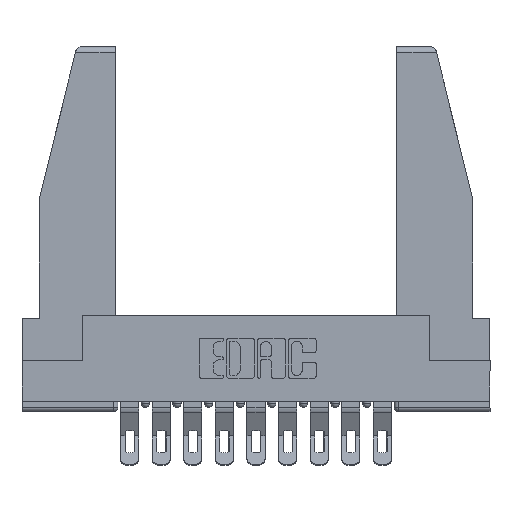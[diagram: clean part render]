
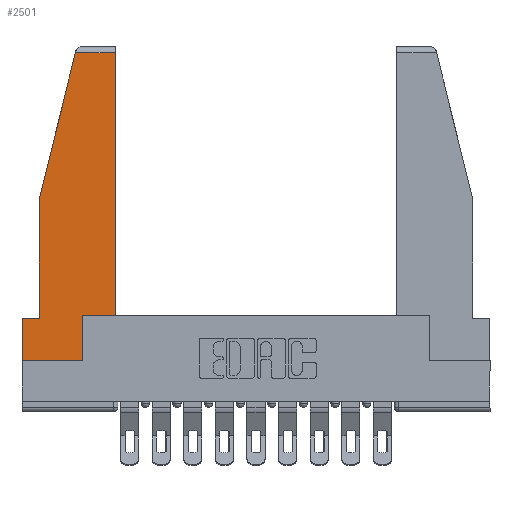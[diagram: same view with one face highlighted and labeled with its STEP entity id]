
A CAD part, top view. The second image highlights one B-rep face of the part: STEP entity #2501.
In plain terms, the highlighted planar face has unit normal (0, 0, 1).
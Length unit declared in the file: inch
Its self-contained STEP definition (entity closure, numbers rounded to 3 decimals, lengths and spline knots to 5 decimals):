
#206 = ORIENTED_EDGE ( 'NONE', *, *, #1486, .T. ) ;
#333 = DIRECTION ( 'NONE',  ( 0., 1., 0. ) ) ;
#355 = CARTESIAN_POINT ( 'NONE',  ( 0.086, 0.8, 0. ) ) ;
#567 = VECTOR ( 'NONE', #10126, 39.37008 ) ;
#826 = LINE ( 'NONE', #355, #5930 ) ;
#1219 = CARTESIAN_POINT ( 'NONE',  ( 0.086, 0.8, 0. ) ) ;
#1256 = CARTESIAN_POINT ( 'NONE',  ( 0.297, 0.223, 0. ) ) ;
#1348 = EDGE_CURVE ( 'NONE', #10210, #10913, #826, .T. ) ;
#1486 = EDGE_CURVE ( 'NONE', #3842, #10258, #7211, .T. ) ;
#1741 = LINE ( 'NONE', #11363, #9174 ) ;
#2501 = ADVANCED_FACE ( 'NONE', ( #2821 ), #6250, .T. ) ;
#2705 = ORIENTED_EDGE ( 'NONE', *, *, #7768, .T. ) ;
#2821 = FACE_OUTER_BOUND ( 'NONE', #9888, .T. ) ;
#2830 = CARTESIAN_POINT ( 'NONE',  ( 0.461, 0.223, 0. ) ) ;
#2843 = AXIS2_PLACEMENT_3D ( 'NONE', #10923, #8651, #14383 ) ;
#2967 = DIRECTION ( 'NONE',  ( 1., 0., 0. ) ) ;
#3550 = DIRECTION ( 'NONE',  ( 1., 0., 0. ) ) ;
#3830 = VERTEX_POINT ( 'NONE', #7760 ) ;
#3842 = VERTEX_POINT ( 'NONE', #7713 ) ;
#3949 = VECTOR ( 'NONE', #11381, 39.37008 ) ;
#4185 = EDGE_CURVE ( 'NONE', #9118, #10560, #7631, .T. ) ;
#4386 = VERTEX_POINT ( 'NONE', #14714 ) ;
#4511 = CARTESIAN_POINT ( 'NONE',  ( 0.461, 1.52, 0. ) ) ;
#5228 = VECTOR ( 'NONE', #333, 39.37008 ) ;
#5352 = EDGE_CURVE ( 'NONE', #10258, #3830, #6695, .T. ) ;
#5438 = ORIENTED_EDGE ( 'NONE', *, *, #5352, .T. ) ;
#5478 = CARTESIAN_POINT ( 'NONE',  ( 0., 0.21, 0. ) ) ;
#5603 = EDGE_CURVE ( 'NONE', #4386, #3842, #9974, .T. ) ;
#5852 = CARTESIAN_POINT ( 'NONE',  ( 0.2636, 1.52, 0. ) ) ;
#5930 = VECTOR ( 'NONE', #13305, 39.37008 ) ;
#6107 = VECTOR ( 'NONE', #2967, 39.37008 ) ;
#6114 = CARTESIAN_POINT ( 'NONE',  ( 0.297, 0., 0. ) ) ;
#6250 = PLANE ( 'NONE',  #2843 ) ;
#6681 = CARTESIAN_POINT ( 'NONE',  ( 0.086, 0.21, 0. ) ) ;
#6695 = LINE ( 'NONE', #6114, #5228 ) ;
#6709 = DIRECTION ( 'NONE',  ( -1., 0., 0. ) ) ;
#6761 = CARTESIAN_POINT ( 'NONE',  ( 0., 0.21, 0. ) ) ;
#7127 = LINE ( 'NONE', #12320, #567 ) ;
#7142 = ORIENTED_EDGE ( 'NONE', *, *, #5603, .T. ) ;
#7211 = LINE ( 'NONE', #7672, #6107 ) ;
#7631 = LINE ( 'NONE', #9430, #13089 ) ;
#7672 = CARTESIAN_POINT ( 'NONE',  ( 0., 0., 0. ) ) ;
#7713 = CARTESIAN_POINT ( 'NONE',  ( 0., 0., 0. ) ) ;
#7760 = CARTESIAN_POINT ( 'NONE',  ( 0.297, 0.223, 0. ) ) ;
#7768 = EDGE_CURVE ( 'NONE', #10560, #10210, #1741, .T. ) ;
#7935 = DIRECTION ( 'NONE',  ( -0.239, -0.971, 0. ) ) ;
#8023 = VECTOR ( 'NONE', #6709, 39.37008 ) ;
#8101 = ORIENTED_EDGE ( 'NONE', *, *, #12726, .T. ) ;
#8182 = VERTEX_POINT ( 'NONE', #2830 ) ;
#8651 = DIRECTION ( 'NONE',  ( 0., 0., 1. ) ) ;
#9118 = VERTEX_POINT ( 'NONE', #4511 ) ;
#9174 = VECTOR ( 'NONE', #7935, 39.37008 ) ;
#9371 = ORIENTED_EDGE ( 'NONE', *, *, #4185, .T. ) ;
#9430 = CARTESIAN_POINT ( 'NONE',  ( 0., 1.52, 0. ) ) ;
#9443 = EDGE_CURVE ( 'NONE', #8182, #9118, #7127, .T. ) ;
#9888 = EDGE_LOOP ( 'NONE', ( #12406, #9371, #2705, #12082, #8101, #7142, #206, #5438, #11670 ) ) ;
#9974 = LINE ( 'NONE', #5478, #3949 ) ;
#10037 = LINE ( 'NONE', #1256, #14045 ) ;
#10126 = DIRECTION ( 'NONE',  ( 0., 1., 0. ) ) ;
#10210 = VERTEX_POINT ( 'NONE', #1219 ) ;
#10258 = VERTEX_POINT ( 'NONE', #10525 ) ;
#10507 = DIRECTION ( 'NONE',  ( -1., 0., 0. ) ) ;
#10525 = CARTESIAN_POINT ( 'NONE',  ( 0.297, 0., 0. ) ) ;
#10560 = VERTEX_POINT ( 'NONE', #5852 ) ;
#10913 = VERTEX_POINT ( 'NONE', #6681 ) ;
#10923 = CARTESIAN_POINT ( 'NONE',  ( 0., 0., 0. ) ) ;
#11363 = CARTESIAN_POINT ( 'NONE',  ( 0.271, 1.55, 0. ) ) ;
#11381 = DIRECTION ( 'NONE',  ( 0., -1., 0. ) ) ;
#11670 = ORIENTED_EDGE ( 'NONE', *, *, #12157, .T. ) ;
#12082 = ORIENTED_EDGE ( 'NONE', *, *, #1348, .T. ) ;
#12157 = EDGE_CURVE ( 'NONE', #3830, #8182, #10037, .T. ) ;
#12320 = CARTESIAN_POINT ( 'NONE',  ( 0.461, 0.223, 0. ) ) ;
#12406 = ORIENTED_EDGE ( 'NONE', *, *, #9443, .T. ) ;
#12726 = EDGE_CURVE ( 'NONE', #10913, #4386, #14921, .T. ) ;
#13089 = VECTOR ( 'NONE', #10507, 39.37008 ) ;
#13305 = DIRECTION ( 'NONE',  ( 0., -1., 0. ) ) ;
#14045 = VECTOR ( 'NONE', #3550, 39.37008 ) ;
#14383 = DIRECTION ( 'NONE',  ( 1., 0., 0. ) ) ;
#14714 = CARTESIAN_POINT ( 'NONE',  ( 0., 0.21, 0. ) ) ;
#14921 = LINE ( 'NONE', #6761, #8023 ) ;
